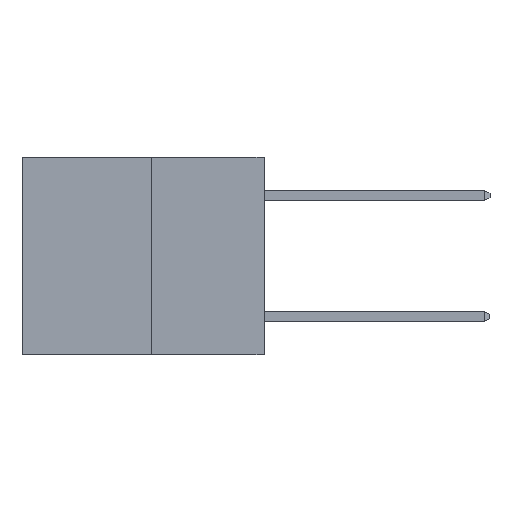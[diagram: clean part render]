
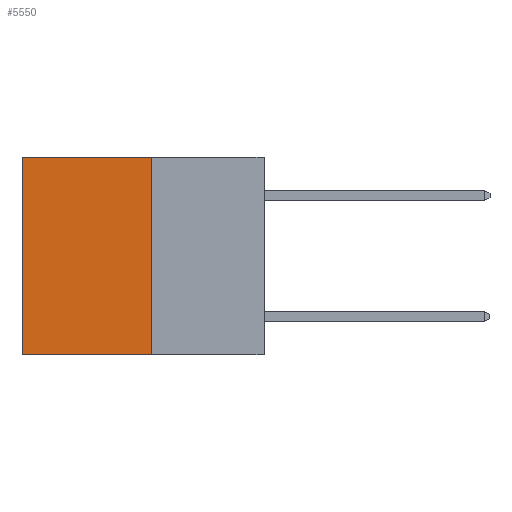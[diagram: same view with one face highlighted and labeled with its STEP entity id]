
A CAD part, left-side view. The second image highlights one B-rep face of the part: STEP entity #5550.
In plain terms, the highlighted planar face has unit normal (-1, 0, 0).
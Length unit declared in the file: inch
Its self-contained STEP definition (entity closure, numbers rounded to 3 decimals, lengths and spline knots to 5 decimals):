
#35 = CARTESIAN_POINT ( 'NONE',  ( 0.3165, 0.28, -0.49 ) ) ;
#156 = DIRECTION ( 'NONE',  ( 0., 1., 0. ) ) ;
#745 = CARTESIAN_POINT ( 'NONE',  ( 0.3165, 0.6, 0. ) ) ;
#1521 = ORIENTED_EDGE ( 'NONE', *, *, #17004, .F. ) ;
#2461 = CARTESIAN_POINT ( 'NONE',  ( 0.3165, 0.28, 0. ) ) ;
#3426 = CARTESIAN_POINT ( 'NONE',  ( 0.3165, 0.6, -0.49 ) ) ;
#3444 = LINE ( 'NONE', #2461, #4335 ) ;
#4123 = VECTOR ( 'NONE', #9817, 39.37008 ) ;
#4335 = VECTOR ( 'NONE', #18137, 39.37008 ) ;
#4890 = VECTOR ( 'NONE', #156, 39.37008 ) ;
#5098 = PLANE ( 'NONE',  #8515 ) ;
#5363 = CARTESIAN_POINT ( 'NONE',  ( 0.3165, 0.28, 0. ) ) ;
#5550 = ADVANCED_FACE ( 'NONE', ( #9981 ), #5098, .F. ) ;
#5768 = DIRECTION ( 'NONE',  ( 0., 0., -1. ) ) ;
#6188 = CARTESIAN_POINT ( 'NONE',  ( 0.3165, 0.28, -0.49 ) ) ;
#6257 = CARTESIAN_POINT ( 'NONE',  ( 0.3165, 0.28, -0.49 ) ) ;
#7289 = DIRECTION ( 'NONE',  ( 1., 0., 0. ) ) ;
#8072 = VERTEX_POINT ( 'NONE', #5363 ) ;
#8269 = CARTESIAN_POINT ( 'NONE',  ( 0.3165, 0.28, -0.49 ) ) ;
#8515 = AXIS2_PLACEMENT_3D ( 'NONE', #35, #7289, #5768 ) ;
#9044 = ORIENTED_EDGE ( 'NONE', *, *, #10899, .T. ) ;
#9817 = DIRECTION ( 'NONE',  ( 0., 0., -1. ) ) ;
#9981 = FACE_OUTER_BOUND ( 'NONE', #10937, .T. ) ;
#10030 = VECTOR ( 'NONE', #16420, 39.37008 ) ;
#10529 = ORIENTED_EDGE ( 'NONE', *, *, #17573, .F. ) ;
#10677 = ORIENTED_EDGE ( 'NONE', *, *, #15563, .T. ) ;
#10899 = EDGE_CURVE ( 'NONE', #13829, #18086, #13465, .T. ) ;
#10937 = EDGE_LOOP ( 'NONE', ( #9044, #1521, #10529, #10677 ) ) ;
#12318 = CARTESIAN_POINT ( 'NONE',  ( 0.3165, 0.6, -0.49 ) ) ;
#13465 = LINE ( 'NONE', #3426, #10030 ) ;
#13666 = VERTEX_POINT ( 'NONE', #6188 ) ;
#13829 = VERTEX_POINT ( 'NONE', #745 ) ;
#14600 = LINE ( 'NONE', #8269, #4123 ) ;
#15563 = EDGE_CURVE ( 'NONE', #8072, #13829, #3444, .T. ) ;
#16420 = DIRECTION ( 'NONE',  ( 0., 0., -1. ) ) ;
#16486 = LINE ( 'NONE', #6257, #4890 ) ;
#17004 = EDGE_CURVE ( 'NONE', #13666, #18086, #16486, .T. ) ;
#17573 = EDGE_CURVE ( 'NONE', #8072, #13666, #14600, .T. ) ;
#18086 = VERTEX_POINT ( 'NONE', #12318 ) ;
#18137 = DIRECTION ( 'NONE',  ( 0., 1., 0. ) ) ;
